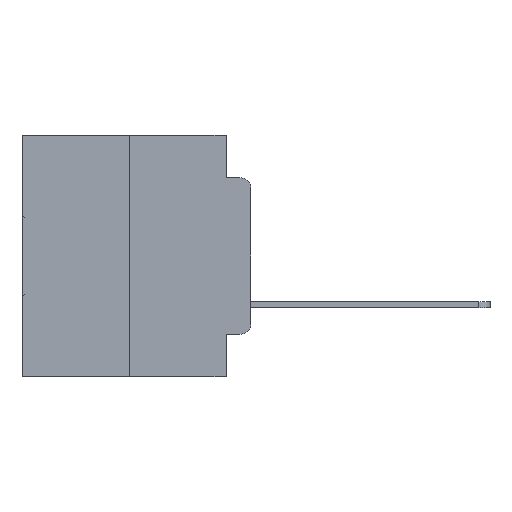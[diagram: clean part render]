
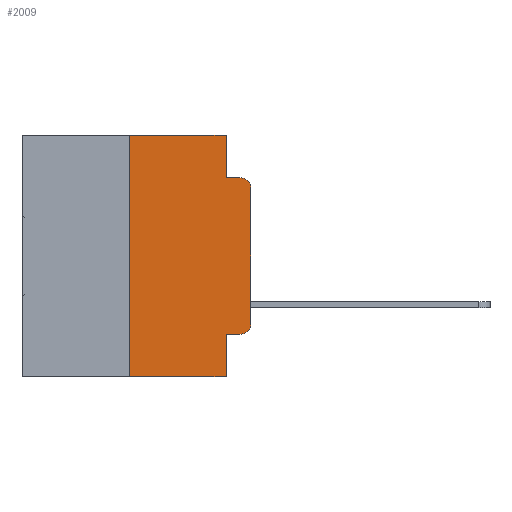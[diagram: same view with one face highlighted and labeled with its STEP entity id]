
A CAD part, left-side view. The second image highlights one B-rep face of the part: STEP entity #2009.
In plain terms, the highlighted planar face has unit normal (-1, 0, 0).
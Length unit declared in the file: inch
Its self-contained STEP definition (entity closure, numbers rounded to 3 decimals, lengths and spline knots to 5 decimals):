
#154 = VECTOR ( 'NONE', #20177, 39.37008 ) ;
#678 = AXIS2_PLACEMENT_3D ( 'NONE', #2398, #19694, #4914 ) ;
#846 = CARTESIAN_POINT ( 'NONE',  ( 0., 0.051, -0.5 ) ) ;
#852 = CARTESIAN_POINT ( 'NONE',  ( 0., 0.02, -0.4115 ) ) ;
#932 = CARTESIAN_POINT ( 'NONE',  ( 0., 0.051, -0.4115 ) ) ;
#940 = LINE ( 'NONE', #29856, #154 ) ;
#970 = VECTOR ( 'NONE', #19511, 39.37008 ) ;
#1260 = AXIS2_PLACEMENT_3D ( 'NONE', #5433, #10396, #27590 ) ;
#1651 = CIRCLE ( 'NONE', #18260, 0.02 ) ;
#2009 = ADVANCED_FACE ( 'NONE', ( #18269 ), #5328, .F. ) ;
#2092 = CARTESIAN_POINT ( 'NONE',  ( 0., 0.02, -0.3915 ) ) ;
#2398 = CARTESIAN_POINT ( 'NONE',  ( 0., 0.02, -0.1085 ) ) ;
#2968 = VERTEX_POINT ( 'NONE', #26076 ) ;
#3698 = VERTEX_POINT ( 'NONE', #21313 ) ;
#4002 = ORIENTED_EDGE ( 'NONE', *, *, #16289, .F. ) ;
#4328 = VERTEX_POINT ( 'NONE', #23858 ) ;
#4431 = VERTEX_POINT ( 'NONE', #24189 ) ;
#4616 = DIRECTION ( 'NONE',  ( 0., 0., -1. ) ) ;
#4914 = DIRECTION ( 'NONE',  ( 0., 0., -1. ) ) ;
#5328 = PLANE ( 'NONE',  #1260 ) ;
#5433 = CARTESIAN_POINT ( 'NONE',  ( 0., 0.473, 0. ) ) ;
#5549 = EDGE_CURVE ( 'NONE', #12079, #16759, #19666, .T. ) ;
#6732 = ORIENTED_EDGE ( 'NONE', *, *, #13819, .F. ) ;
#7248 = EDGE_CURVE ( 'NONE', #12079, #31051, #8452, .T. ) ;
#7673 = EDGE_CURVE ( 'NONE', #4431, #31051, #940, .T. ) ;
#8452 = LINE ( 'NONE', #31596, #970 ) ;
#8898 = EDGE_CURVE ( 'NONE', #4431, #3698, #30081, .T. ) ;
#9043 = VECTOR ( 'NONE', #29460, 39.37008 ) ;
#9362 = CIRCLE ( 'NONE', #678, 0.02 ) ;
#9414 = ORIENTED_EDGE ( 'NONE', *, *, #17106, .T. ) ;
#9791 = LINE ( 'NONE', #19663, #9043 ) ;
#9799 = VECTOR ( 'NONE', #25271, 39.37008 ) ;
#10065 = VECTOR ( 'NONE', #30054, 39.37008 ) ;
#10396 = DIRECTION ( 'NONE',  ( 1., 0., 0. ) ) ;
#10810 = LINE ( 'NONE', #15397, #10065 ) ;
#10930 = CARTESIAN_POINT ( 'NONE',  ( 0., 0.02, -0.0885 ) ) ;
#10941 = DIRECTION ( 'NONE',  ( 0., -1., 0. ) ) ;
#11670 = LINE ( 'NONE', #28375, #17459 ) ;
#12079 = VERTEX_POINT ( 'NONE', #31641 ) ;
#12153 = EDGE_CURVE ( 'NONE', #26295, #4328, #9791, .T. ) ;
#12784 = DIRECTION ( 'NONE',  ( 0., -1., 0. ) ) ;
#12862 = CARTESIAN_POINT ( 'NONE',  ( 0., 0.25, 0. ) ) ;
#13080 = VECTOR ( 'NONE', #10941, 39.37008 ) ;
#13819 = EDGE_CURVE ( 'NONE', #4328, #27004, #21594, .T. ) ;
#15003 = VECTOR ( 'NONE', #12784, 39.37008 ) ;
#15247 = CARTESIAN_POINT ( 'NONE',  ( 0., 0.051, -0.0885 ) ) ;
#15397 = CARTESIAN_POINT ( 'NONE',  ( 0., 0.473, 0. ) ) ;
#15438 = EDGE_CURVE ( 'NONE', #2968, #27004, #9362, .T. ) ;
#16289 = EDGE_CURVE ( 'NONE', #3698, #26295, #10810, .T. ) ;
#16695 = EDGE_LOOP ( 'NONE', ( #9414, #24056, #6732, #22161, #4002, #17112, #27498, #31237, #27886, #30125 ) ) ;
#16759 = VERTEX_POINT ( 'NONE', #852 ) ;
#17106 = EDGE_CURVE ( 'NONE', #17936, #2968, #11670, .T. ) ;
#17112 = ORIENTED_EDGE ( 'NONE', *, *, #8898, .F. ) ;
#17459 = VECTOR ( 'NONE', #30785, 39.37008 ) ;
#17936 = VERTEX_POINT ( 'NONE', #19783 ) ;
#18260 = AXIS2_PLACEMENT_3D ( 'NONE', #2092, #19399, #4616 ) ;
#18269 = FACE_OUTER_BOUND ( 'NONE', #16695, .T. ) ;
#19399 = DIRECTION ( 'NONE',  ( -1., 0., 0. ) ) ;
#19511 = DIRECTION ( 'NONE',  ( 0., 0., -1. ) ) ;
#19663 = CARTESIAN_POINT ( 'NONE',  ( 0., 0.051, 0. ) ) ;
#19666 = LINE ( 'NONE', #932, #13080 ) ;
#19694 = DIRECTION ( 'NONE',  ( -1., 0., 0. ) ) ;
#19783 = CARTESIAN_POINT ( 'NONE',  ( 0., 0., -0.3915 ) ) ;
#20177 = DIRECTION ( 'NONE',  ( 0., -1., 0. ) ) ;
#21313 = CARTESIAN_POINT ( 'NONE',  ( 0., 0.25, 0. ) ) ;
#21594 = LINE ( 'NONE', #15247, #15003 ) ;
#22161 = ORIENTED_EDGE ( 'NONE', *, *, #12153, .F. ) ;
#23858 = CARTESIAN_POINT ( 'NONE',  ( 0., 0.051, -0.0885 ) ) ;
#24056 = ORIENTED_EDGE ( 'NONE', *, *, #15438, .T. ) ;
#24189 = CARTESIAN_POINT ( 'NONE',  ( 0., 0.25, -0.5 ) ) ;
#25271 = DIRECTION ( 'NONE',  ( 0., 0., 1. ) ) ;
#26076 = CARTESIAN_POINT ( 'NONE',  ( 0., 0., -0.1085 ) ) ;
#26295 = VERTEX_POINT ( 'NONE', #30339 ) ;
#27004 = VERTEX_POINT ( 'NONE', #10930 ) ;
#27498 = ORIENTED_EDGE ( 'NONE', *, *, #7673, .T. ) ;
#27590 = DIRECTION ( 'NONE',  ( 0., 0., -1. ) ) ;
#27886 = ORIENTED_EDGE ( 'NONE', *, *, #5549, .T. ) ;
#28375 = CARTESIAN_POINT ( 'NONE',  ( 0., 0., 0. ) ) ;
#29460 = DIRECTION ( 'NONE',  ( 0., 0., -1. ) ) ;
#29856 = CARTESIAN_POINT ( 'NONE',  ( 0., 0.473, -0.5 ) ) ;
#30054 = DIRECTION ( 'NONE',  ( 0., -1., 0. ) ) ;
#30081 = LINE ( 'NONE', #12862, #9799 ) ;
#30125 = ORIENTED_EDGE ( 'NONE', *, *, #30809, .T. ) ;
#30339 = CARTESIAN_POINT ( 'NONE',  ( 0., 0.051, 0. ) ) ;
#30785 = DIRECTION ( 'NONE',  ( 0., 0., 1. ) ) ;
#30809 = EDGE_CURVE ( 'NONE', #16759, #17936, #1651, .T. ) ;
#31051 = VERTEX_POINT ( 'NONE', #846 ) ;
#31237 = ORIENTED_EDGE ( 'NONE', *, *, #7248, .F. ) ;
#31596 = CARTESIAN_POINT ( 'NONE',  ( 0., 0.051, 0. ) ) ;
#31641 = CARTESIAN_POINT ( 'NONE',  ( 0., 0.051, -0.4115 ) ) ;
